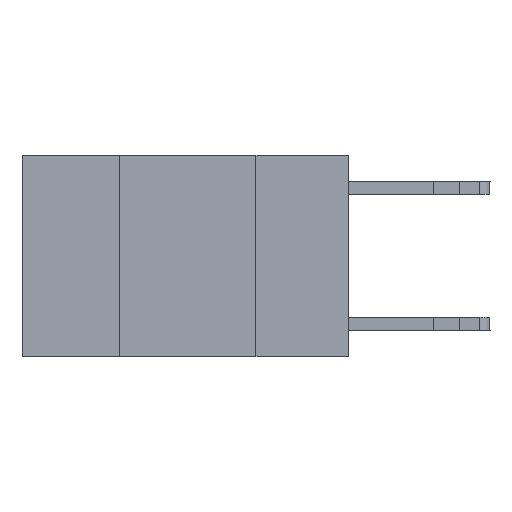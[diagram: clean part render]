
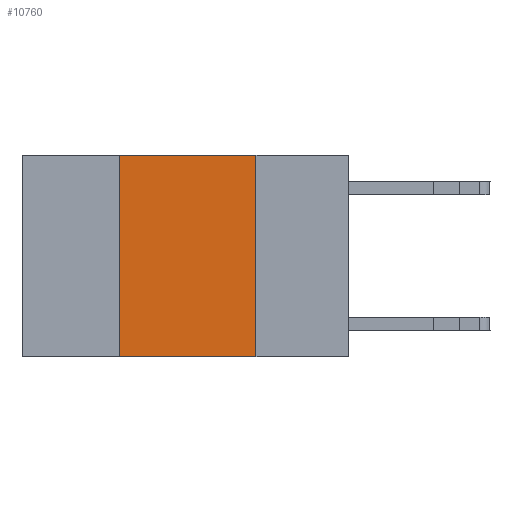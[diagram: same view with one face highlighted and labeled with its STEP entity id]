
A CAD part, left-side view. The second image highlights one B-rep face of the part: STEP entity #10760.
In plain terms, the highlighted planar face has unit normal (-1, 0, 0).
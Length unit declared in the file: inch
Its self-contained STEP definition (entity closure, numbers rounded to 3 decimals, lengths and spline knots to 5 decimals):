
#179 = FACE_OUTER_BOUND ( 'NONE', #12861, .T. ) ;
#369 = DIRECTION ( 'NONE',  ( 0., -1., 0. ) ) ;
#668 = DIRECTION ( 'NONE',  ( 0., 0., 1. ) ) ;
#693 = ORIENTED_EDGE ( 'NONE', *, *, #11565, .F. ) ;
#1234 = VERTEX_POINT ( 'NONE', #1424 ) ;
#1369 = VECTOR ( 'NONE', #369, 39.37008 ) ;
#1424 = CARTESIAN_POINT ( 'NONE',  ( 0., 0.42, -0.37 ) ) ;
#1508 = VERTEX_POINT ( 'NONE', #12358 ) ;
#1923 = LINE ( 'NONE', #13321, #3632 ) ;
#1940 = EDGE_CURVE ( 'NONE', #1234, #1508, #7999, .T. ) ;
#2139 = DIRECTION ( 'NONE',  ( 0., -1., 0. ) ) ;
#2910 = EDGE_CURVE ( 'NONE', #10739, #6324, #6016, .T. ) ;
#3632 = VECTOR ( 'NONE', #668, 39.37008 ) ;
#4351 = ORIENTED_EDGE ( 'NONE', *, *, #9235, .F. ) ;
#5340 = CARTESIAN_POINT ( 'NONE',  ( 0., 0.6, 0. ) ) ;
#5397 = DIRECTION ( 'NONE',  ( 0., 0., -1. ) ) ;
#5847 = ORIENTED_EDGE ( 'NONE', *, *, #1940, .T. ) ;
#6016 = LINE ( 'NONE', #7057, #1369 ) ;
#6052 = ORIENTED_EDGE ( 'NONE', *, *, #2910, .F. ) ;
#6324 = VERTEX_POINT ( 'NONE', #6443 ) ;
#6443 = CARTESIAN_POINT ( 'NONE',  ( 0., 0.17, 0. ) ) ;
#7057 = CARTESIAN_POINT ( 'NONE',  ( 0., 0.6, 0. ) ) ;
#7542 = LINE ( 'NONE', #13281, #10033 ) ;
#7969 = CARTESIAN_POINT ( 'NONE',  ( 0., 0.42, 0. ) ) ;
#7999 = LINE ( 'NONE', #11151, #12281 ) ;
#8595 = AXIS2_PLACEMENT_3D ( 'NONE', #5340, #9104, #9875 ) ;
#9104 = DIRECTION ( 'NONE',  ( 1., 0., 0. ) ) ;
#9235 = EDGE_CURVE ( 'NONE', #6324, #1508, #7542, .T. ) ;
#9875 = DIRECTION ( 'NONE',  ( 0., 0., -1. ) ) ;
#10033 = VECTOR ( 'NONE', #5397, 39.37008 ) ;
#10739 = VERTEX_POINT ( 'NONE', #7969 ) ;
#10760 = ADVANCED_FACE ( 'NONE', ( #179 ), #11065, .F. ) ;
#11065 = PLANE ( 'NONE',  #8595 ) ;
#11151 = CARTESIAN_POINT ( 'NONE',  ( 0., 0.6, -0.37 ) ) ;
#11565 = EDGE_CURVE ( 'NONE', #1234, #10739, #1923, .T. ) ;
#12281 = VECTOR ( 'NONE', #2139, 39.37008 ) ;
#12358 = CARTESIAN_POINT ( 'NONE',  ( 0., 0.17, -0.37 ) ) ;
#12861 = EDGE_LOOP ( 'NONE', ( #4351, #6052, #693, #5847 ) ) ;
#13281 = CARTESIAN_POINT ( 'NONE',  ( 0., 0.17, 0. ) ) ;
#13321 = CARTESIAN_POINT ( 'NONE',  ( 0., 0.42, 0. ) ) ;
